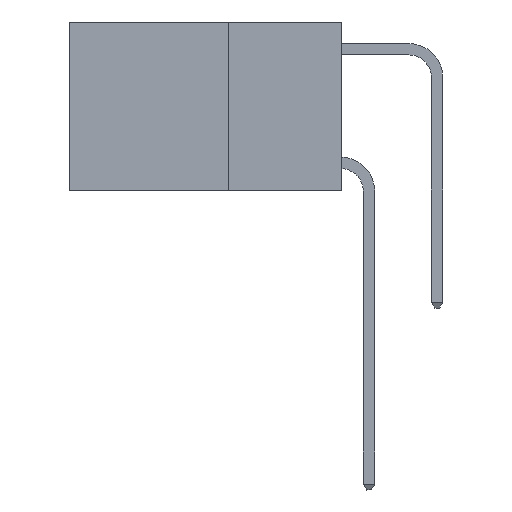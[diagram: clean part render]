
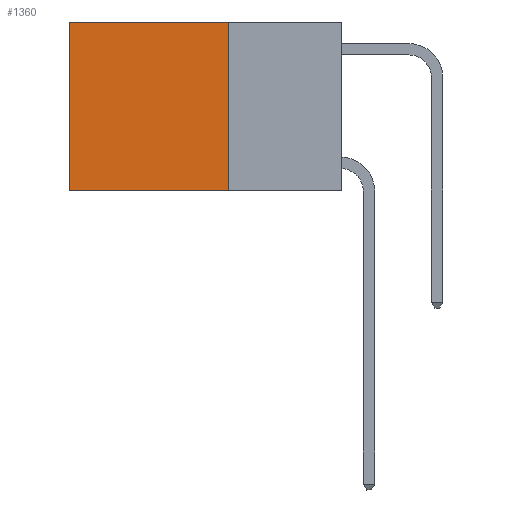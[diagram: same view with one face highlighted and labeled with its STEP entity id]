
A CAD part, left-side view. The second image highlights one B-rep face of the part: STEP entity #1360.
In plain terms, the highlighted planar face has unit normal (-1, 0, 0).
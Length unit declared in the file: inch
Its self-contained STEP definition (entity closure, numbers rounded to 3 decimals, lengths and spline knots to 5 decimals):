
#224 = VERTEX_POINT ( 'NONE', #8396 ) ;
#529 = DIRECTION ( 'NONE',  ( 0., 0., -1. ) ) ;
#778 = VECTOR ( 'NONE', #2728, 39.37008 ) ;
#1360 = ADVANCED_FACE ( 'NONE', ( #3970 ), #11985, .F. ) ;
#1935 = EDGE_CURVE ( 'NONE', #5274, #224, #3518, .T. ) ;
#2112 = DIRECTION ( 'NONE',  ( 0., 0., -1. ) ) ;
#2438 = ORIENTED_EDGE ( 'NONE', *, *, #3380, .T. ) ;
#2728 = DIRECTION ( 'NONE',  ( 0., 1., 0. ) ) ;
#2730 = CARTESIAN_POINT ( 'NONE',  ( 0.2625, 0.25, -0.37 ) ) ;
#3380 = EDGE_CURVE ( 'NONE', #8367, #224, #15054, .T. ) ;
#3518 = LINE ( 'NONE', #5201, #778 ) ;
#3580 = CARTESIAN_POINT ( 'NONE',  ( 0.2625, 0.25, 0. ) ) ;
#3722 = EDGE_CURVE ( 'NONE', #9460, #8367, #13233, .T. ) ;
#3970 = FACE_OUTER_BOUND ( 'NONE', #4974, .T. ) ;
#4560 = EDGE_CURVE ( 'NONE', #9460, #5274, #11681, .T. ) ;
#4921 = CARTESIAN_POINT ( 'NONE',  ( 0.2625, 0.25, 0. ) ) ;
#4974 = EDGE_LOOP ( 'NONE', ( #2438, #11405, #14055, #5246 ) ) ;
#5201 = CARTESIAN_POINT ( 'NONE',  ( 0.2625, 0.25, -0.37 ) ) ;
#5246 = ORIENTED_EDGE ( 'NONE', *, *, #3722, .T. ) ;
#5274 = VERTEX_POINT ( 'NONE', #2730 ) ;
#5665 = DIRECTION ( 'NONE',  ( 0., 1., 0. ) ) ;
#6560 = CARTESIAN_POINT ( 'NONE',  ( 0.2625, 0.6, 0. ) ) ;
#8367 = VERTEX_POINT ( 'NONE', #8982 ) ;
#8396 = CARTESIAN_POINT ( 'NONE',  ( 0.2625, 0.6, -0.37 ) ) ;
#8982 = CARTESIAN_POINT ( 'NONE',  ( 0.2625, 0.6, 0. ) ) ;
#9460 = VERTEX_POINT ( 'NONE', #3580 ) ;
#10896 = DIRECTION ( 'NONE',  ( 1., 0., 0. ) ) ;
#10990 = VECTOR ( 'NONE', #529, 39.37008 ) ;
#11405 = ORIENTED_EDGE ( 'NONE', *, *, #1935, .F. ) ;
#11681 = LINE ( 'NONE', #12643, #13753 ) ;
#11985 = PLANE ( 'NONE',  #13306 ) ;
#12091 = DIRECTION ( 'NONE',  ( 0., 0., -1. ) ) ;
#12643 = CARTESIAN_POINT ( 'NONE',  ( 0.2625, 0.25, 0. ) ) ;
#13233 = LINE ( 'NONE', #13558, #14521 ) ;
#13306 = AXIS2_PLACEMENT_3D ( 'NONE', #4921, #10896, #12091 ) ;
#13558 = CARTESIAN_POINT ( 'NONE',  ( 0.2625, 0.25, 0. ) ) ;
#13753 = VECTOR ( 'NONE', #2112, 39.37008 ) ;
#14055 = ORIENTED_EDGE ( 'NONE', *, *, #4560, .F. ) ;
#14521 = VECTOR ( 'NONE', #5665, 39.37008 ) ;
#15054 = LINE ( 'NONE', #6560, #10990 ) ;
